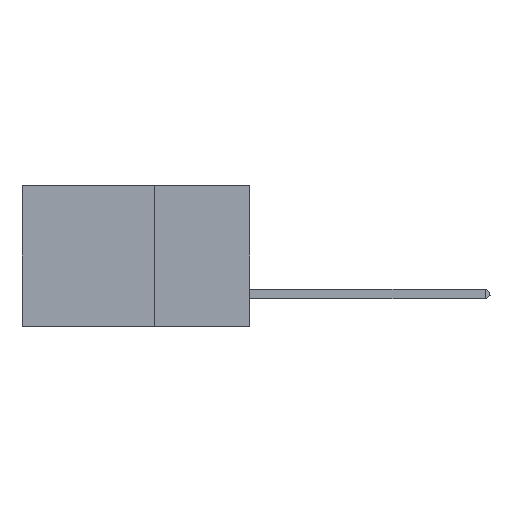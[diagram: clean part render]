
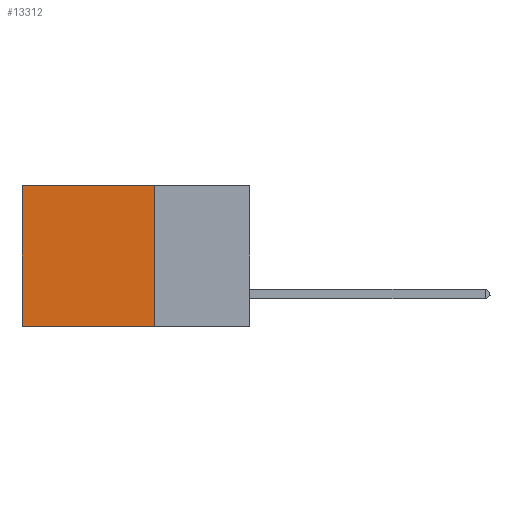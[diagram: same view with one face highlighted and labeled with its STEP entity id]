
A CAD part, left-side view. The second image highlights one B-rep face of the part: STEP entity #13312.
In plain terms, the highlighted planar face has unit normal (-1, 0, 0).
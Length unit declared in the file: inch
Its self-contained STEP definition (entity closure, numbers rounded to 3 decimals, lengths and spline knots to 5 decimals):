
#149 = FACE_OUTER_BOUND ( 'NONE', #4838, .T. ) ;
#267 = CARTESIAN_POINT ( 'NONE',  ( 0.2875, 0.6, -0.37 ) ) ;
#1119 = EDGE_CURVE ( 'NONE', #21712, #21284, #12514, .T. ) ;
#1213 = VERTEX_POINT ( 'NONE', #15318 ) ;
#1937 = VERTEX_POINT ( 'NONE', #13452 ) ;
#2174 = CARTESIAN_POINT ( 'NONE',  ( 0.2875, 0.25, 0. ) ) ;
#2297 = VECTOR ( 'NONE', #16456, 39.37008 ) ;
#2711 = ORIENTED_EDGE ( 'NONE', *, *, #3774, .F. ) ;
#3774 = EDGE_CURVE ( 'NONE', #1937, #21284, #12665, .T. ) ;
#4596 = AXIS2_PLACEMENT_3D ( 'NONE', #5007, #10718, #17652 ) ;
#4838 = EDGE_LOOP ( 'NONE', ( #16988, #2711, #16838, #22677 ) ) ;
#5007 = CARTESIAN_POINT ( 'NONE',  ( 0.2875, 0.25, 0. ) ) ;
#5801 = CARTESIAN_POINT ( 'NONE',  ( 0.2875, 0.25, 0. ) ) ;
#7159 = PLANE ( 'NONE',  #4596 ) ;
#7749 = VECTOR ( 'NONE', #13058, 39.37008 ) ;
#8640 = EDGE_CURVE ( 'NONE', #1213, #1937, #14803, .T. ) ;
#8660 = CARTESIAN_POINT ( 'NONE',  ( 0.2875, 0.6, 0. ) ) ;
#10572 = VECTOR ( 'NONE', #14213, 39.37008 ) ;
#10718 = DIRECTION ( 'NONE',  ( 1., 0., 0. ) ) ;
#12287 = CARTESIAN_POINT ( 'NONE',  ( 0.2875, 0.25, -0.37 ) ) ;
#12514 = LINE ( 'NONE', #17865, #10572 ) ;
#12665 = LINE ( 'NONE', #12287, #18065 ) ;
#13058 = DIRECTION ( 'NONE',  ( 0., 1., 0. ) ) ;
#13312 = ADVANCED_FACE ( 'NONE', ( #149 ), #7159, .F. ) ;
#13452 = CARTESIAN_POINT ( 'NONE',  ( 0.2875, 0.25, -0.37 ) ) ;
#13943 = DIRECTION ( 'NONE',  ( 0., 1., 0. ) ) ;
#14213 = DIRECTION ( 'NONE',  ( 0., 0., -1. ) ) ;
#14803 = LINE ( 'NONE', #5801, #2297 ) ;
#15318 = CARTESIAN_POINT ( 'NONE',  ( 0.2875, 0.25, 0. ) ) ;
#16456 = DIRECTION ( 'NONE',  ( 0., 0., -1. ) ) ;
#16838 = ORIENTED_EDGE ( 'NONE', *, *, #8640, .F. ) ;
#16988 = ORIENTED_EDGE ( 'NONE', *, *, #1119, .T. ) ;
#17652 = DIRECTION ( 'NONE',  ( 0., 0., -1. ) ) ;
#17865 = CARTESIAN_POINT ( 'NONE',  ( 0.2875, 0.6, 0. ) ) ;
#18065 = VECTOR ( 'NONE', #13943, 39.37008 ) ;
#21284 = VERTEX_POINT ( 'NONE', #267 ) ;
#21712 = VERTEX_POINT ( 'NONE', #8660 ) ;
#22205 = LINE ( 'NONE', #2174, #7749 ) ;
#22677 = ORIENTED_EDGE ( 'NONE', *, *, #23177, .T. ) ;
#23177 = EDGE_CURVE ( 'NONE', #1213, #21712, #22205, .T. ) ;
